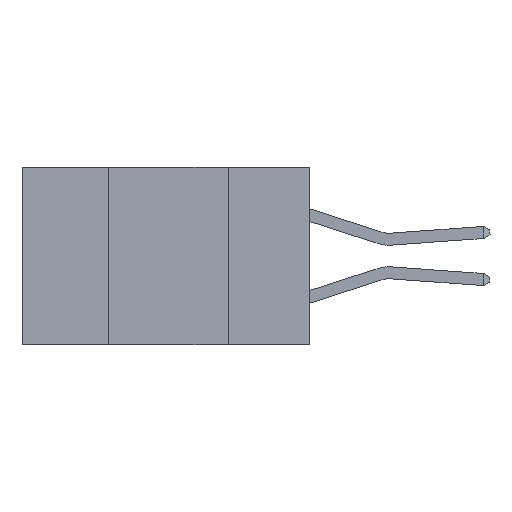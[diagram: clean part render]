
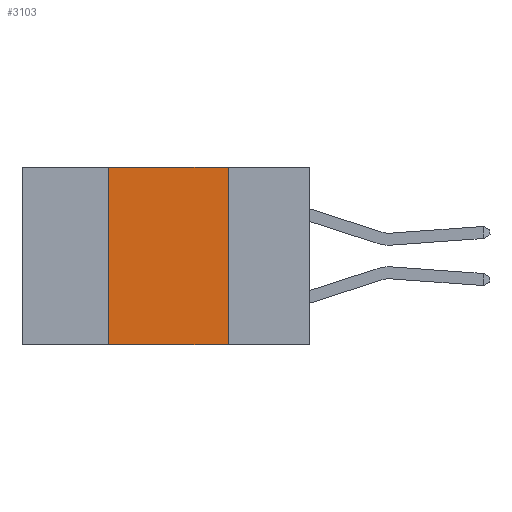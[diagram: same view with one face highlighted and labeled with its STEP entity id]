
A CAD part, left-side view. The second image highlights one B-rep face of the part: STEP entity #3103.
In plain terms, the highlighted planar face has unit normal (-1, 0, 0).
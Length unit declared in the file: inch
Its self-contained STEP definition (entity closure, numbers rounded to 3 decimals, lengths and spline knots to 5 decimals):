
#1149 = EDGE_CURVE ( 'NONE', #12978, #3324, #7210, .T. ) ;
#1239 = EDGE_CURVE ( 'NONE', #2382, #9875, #13567, .T. ) ;
#1459 = VECTOR ( 'NONE', #2471, 39.37008 ) ;
#1857 = CARTESIAN_POINT ( 'NONE',  ( 0., 0.42, -0.37 ) ) ;
#1941 = EDGE_CURVE ( 'NONE', #9875, #12978, #10528, .T. ) ;
#2382 = VERTEX_POINT ( 'NONE', #1857 ) ;
#2471 = DIRECTION ( 'NONE',  ( 0., -1., 0. ) ) ;
#2754 = VECTOR ( 'NONE', #5809, 39.37008 ) ;
#3052 = CARTESIAN_POINT ( 'NONE',  ( 0., 0.17, -0.37 ) ) ;
#3103 = ADVANCED_FACE ( 'NONE', ( #7514 ), #3110, .F. ) ;
#3110 = PLANE ( 'NONE',  #14092 ) ;
#3324 = VERTEX_POINT ( 'NONE', #3052 ) ;
#3775 = ORIENTED_EDGE ( 'NONE', *, *, #1941, .F. ) ;
#4629 = CARTESIAN_POINT ( 'NONE',  ( 0., 0.42, 0. ) ) ;
#5618 = CARTESIAN_POINT ( 'NONE',  ( 0., 0.17, 0. ) ) ;
#5809 = DIRECTION ( 'NONE',  ( 0., -1., 0. ) ) ;
#6322 = CARTESIAN_POINT ( 'NONE',  ( 0., 0.17, 0. ) ) ;
#6607 = ORIENTED_EDGE ( 'NONE', *, *, #1149, .F. ) ;
#6856 = VECTOR ( 'NONE', #13020, 39.37008 ) ;
#7210 = LINE ( 'NONE', #5618, #6856 ) ;
#7514 = FACE_OUTER_BOUND ( 'NONE', #7855, .T. ) ;
#7761 = VECTOR ( 'NONE', #12515, 39.37008 ) ;
#7855 = EDGE_LOOP ( 'NONE', ( #6607, #3775, #9988, #13746 ) ) ;
#8083 = CARTESIAN_POINT ( 'NONE',  ( 0., 0.6, -0.37 ) ) ;
#9299 = DIRECTION ( 'NONE',  ( 0., 0., -1. ) ) ;
#9471 = CARTESIAN_POINT ( 'NONE',  ( 0., 0.6, 0. ) ) ;
#9875 = VERTEX_POINT ( 'NONE', #4629 ) ;
#9988 = ORIENTED_EDGE ( 'NONE', *, *, #1239, .F. ) ;
#10049 = DIRECTION ( 'NONE',  ( 1., 0., 0. ) ) ;
#10528 = LINE ( 'NONE', #13930, #1459 ) ;
#11632 = LINE ( 'NONE', #8083, #2754 ) ;
#12515 = DIRECTION ( 'NONE',  ( 0., 0., 1. ) ) ;
#12978 = VERTEX_POINT ( 'NONE', #6322 ) ;
#13020 = DIRECTION ( 'NONE',  ( 0., 0., -1. ) ) ;
#13567 = LINE ( 'NONE', #14640, #7761 ) ;
#13746 = ORIENTED_EDGE ( 'NONE', *, *, #14529, .T. ) ;
#13930 = CARTESIAN_POINT ( 'NONE',  ( 0., 0.6, 0. ) ) ;
#14092 = AXIS2_PLACEMENT_3D ( 'NONE', #9471, #10049, #9299 ) ;
#14529 = EDGE_CURVE ( 'NONE', #2382, #3324, #11632, .T. ) ;
#14640 = CARTESIAN_POINT ( 'NONE',  ( 0., 0.42, 0. ) ) ;
